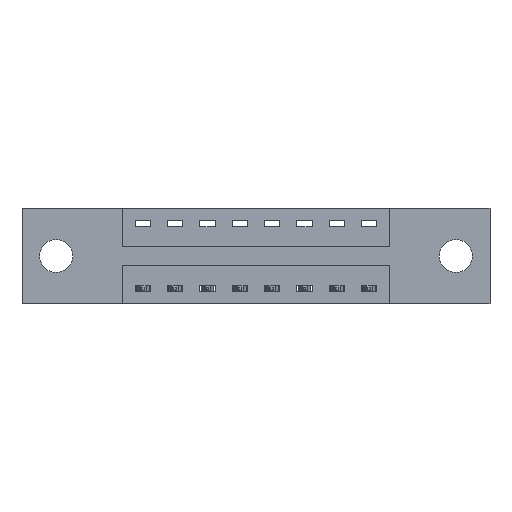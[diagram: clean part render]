
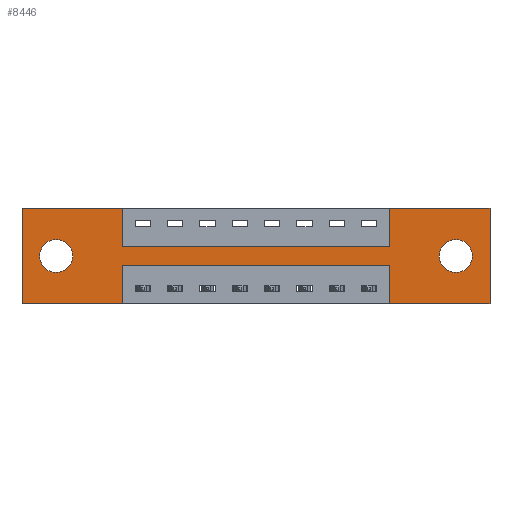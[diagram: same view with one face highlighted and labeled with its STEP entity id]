
A CAD part, front view. The second image highlights one B-rep face of the part: STEP entity #8446.
In plain terms, the highlighted planar face has unit normal (0, -1, 0).
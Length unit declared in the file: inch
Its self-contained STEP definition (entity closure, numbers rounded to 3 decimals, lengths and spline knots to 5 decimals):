
#36 = LINE ( 'NONE', #4405, #9114 ) ;
#68 = CARTESIAN_POINT ( 'NONE',  ( 0.3875, 0., -0.37 ) ) ;
#102 = VECTOR ( 'NONE', #4733, 39.37008 ) ;
#180 = VERTEX_POINT ( 'NONE', #5444 ) ;
#220 = LINE ( 'NONE', #68, #4136 ) ;
#350 = AXIS2_PLACEMENT_3D ( 'NONE', #5021, #8691, #3470 ) ;
#361 = EDGE_CURVE ( 'NONE', #2038, #2089, #7984, .T. ) ;
#451 = CARTESIAN_POINT ( 'NONE',  ( 0.1325, 0., -0.185 ) ) ;
#461 = VECTOR ( 'NONE', #2829, 39.37008 ) ;
#478 = EDGE_CURVE ( 'NONE', #9548, #180, #2171, .T. ) ;
#603 = VERTEX_POINT ( 'NONE', #5477 ) ;
#650 = EDGE_CURVE ( 'NONE', #9427, #603, #4993, .T. ) ;
#817 = CARTESIAN_POINT ( 'NONE',  ( 1.6775, 0., -0.185 ) ) ;
#1143 = VERTEX_POINT ( 'NONE', #4393 ) ;
#1163 = VERTEX_POINT ( 'NONE', #2121 ) ;
#1198 = CARTESIAN_POINT ( 'NONE',  ( 0., 0., -0.37 ) ) ;
#1335 = VECTOR ( 'NONE', #1476, 39.37008 ) ;
#1385 = CARTESIAN_POINT ( 'NONE',  ( 0., 0., 0. ) ) ;
#1429 = LINE ( 'NONE', #1385, #2047 ) ;
#1476 = DIRECTION ( 'NONE',  ( 0., 0., 1. ) ) ;
#1690 = VECTOR ( 'NONE', #2498, 39.37008 ) ;
#1725 = EDGE_LOOP ( 'NONE', ( #2457, #5234, #5663, #4398, #7138, #2356, #2877, #5528, #3506, #6196, #2540, #4841 ) ) ;
#1745 = VERTEX_POINT ( 'NONE', #7530 ) ;
#1828 = DIRECTION ( 'NONE',  ( 0., 0., -1. ) ) ;
#1904 = EDGE_CURVE ( 'NONE', #2089, #7087, #1429, .T. ) ;
#1927 = DIRECTION ( 'NONE',  ( 0., 0., 1. ) ) ;
#1958 = CARTESIAN_POINT ( 'NONE',  ( 1.6775, 0., -0.185 ) ) ;
#2038 = VERTEX_POINT ( 'NONE', #8992 ) ;
#2047 = VECTOR ( 'NONE', #7213, 39.37008 ) ;
#2089 = VERTEX_POINT ( 'NONE', #2553 ) ;
#2121 = CARTESIAN_POINT ( 'NONE',  ( 0.3875, 0., -0.37 ) ) ;
#2154 = EDGE_CURVE ( 'NONE', #180, #9548, #8745, .T. ) ;
#2171 = CIRCLE ( 'NONE', #8862, 0.064 ) ;
#2196 = DIRECTION ( 'NONE',  ( 0., -1., 0. ) ) ;
#2202 = VERTEX_POINT ( 'NONE', #2324 ) ;
#2206 = EDGE_CURVE ( 'NONE', #1143, #1745, #7455, .T. ) ;
#2324 = CARTESIAN_POINT ( 'NONE',  ( 1.81, 0., -0.37 ) ) ;
#2356 = ORIENTED_EDGE ( 'NONE', *, *, #1904, .F. ) ;
#2402 = AXIS2_PLACEMENT_3D ( 'NONE', #2970, #2196, #3796 ) ;
#2457 = ORIENTED_EDGE ( 'NONE', *, *, #4424, .F. ) ;
#2498 = DIRECTION ( 'NONE',  ( 1., 0., 0. ) ) ;
#2540 = ORIENTED_EDGE ( 'NONE', *, *, #4110, .F. ) ;
#2550 = LINE ( 'NONE', #9058, #5057 ) ;
#2553 = CARTESIAN_POINT ( 'NONE',  ( 1.4225, 0., 0. ) ) ;
#2775 = CARTESIAN_POINT ( 'NONE',  ( 1.81, 0., 0. ) ) ;
#2789 = VECTOR ( 'NONE', #8170, 39.37008 ) ;
#2829 = DIRECTION ( 'NONE',  ( 1., 0., 0. ) ) ;
#2877 = ORIENTED_EDGE ( 'NONE', *, *, #361, .F. ) ;
#2970 = CARTESIAN_POINT ( 'NONE',  ( 0., 0., -0.37 ) ) ;
#3041 = CARTESIAN_POINT ( 'NONE',  ( 1.4225, 0., -0.37 ) ) ;
#3123 = FACE_BOUND ( 'NONE', #6140, .T. ) ;
#3143 = ORIENTED_EDGE ( 'NONE', *, *, #2154, .T. ) ;
#3180 = CARTESIAN_POINT ( 'NONE',  ( 0., 0., 0. ) ) ;
#3295 = VERTEX_POINT ( 'NONE', #7139 ) ;
#3379 = LINE ( 'NONE', #6351, #6616 ) ;
#3470 = DIRECTION ( 'NONE',  ( 0., 0., 1. ) ) ;
#3506 = ORIENTED_EDGE ( 'NONE', *, *, #5926, .F. ) ;
#3557 = VECTOR ( 'NONE', #7533, 39.37008 ) ;
#3655 = FACE_OUTER_BOUND ( 'NONE', #1725, .T. ) ;
#3781 = ORIENTED_EDGE ( 'NONE', *, *, #650, .T. ) ;
#3796 = DIRECTION ( 'NONE',  ( 0., 0., -1. ) ) ;
#3813 = VERTEX_POINT ( 'NONE', #6074 ) ;
#3902 = LINE ( 'NONE', #3180, #461 ) ;
#4110 = EDGE_CURVE ( 'NONE', #4231, #3295, #5169, .T. ) ;
#4136 = VECTOR ( 'NONE', #4541, 39.37008 ) ;
#4187 = EDGE_LOOP ( 'NONE', ( #4521, #3781 ) ) ;
#4223 = VECTOR ( 'NONE', #4558, 39.37008 ) ;
#4231 = VERTEX_POINT ( 'NONE', #1198 ) ;
#4342 = CARTESIAN_POINT ( 'NONE',  ( 0.3875, 0., -0.15 ) ) ;
#4378 = CARTESIAN_POINT ( 'NONE',  ( 1.4225, 0., 0. ) ) ;
#4393 = CARTESIAN_POINT ( 'NONE',  ( 1.4225, 0., -0.22 ) ) ;
#4398 = ORIENTED_EDGE ( 'NONE', *, *, #8608, .F. ) ;
#4405 = CARTESIAN_POINT ( 'NONE',  ( 1.81, 0., 0. ) ) ;
#4424 = EDGE_CURVE ( 'NONE', #1745, #1163, #220, .T. ) ;
#4472 = VERTEX_POINT ( 'NONE', #3041 ) ;
#4521 = ORIENTED_EDGE ( 'NONE', *, *, #8176, .T. ) ;
#4541 = DIRECTION ( 'NONE',  ( 0., 0., -1. ) ) ;
#4558 = DIRECTION ( 'NONE',  ( -1., 0., 0. ) ) ;
#4733 = DIRECTION ( 'NONE',  ( -1., 0., 0. ) ) ;
#4841 = ORIENTED_EDGE ( 'NONE', *, *, #8205, .F. ) ;
#4993 = CIRCLE ( 'NONE', #350, 0.064 ) ;
#5021 = CARTESIAN_POINT ( 'NONE',  ( 0.1325, 0., -0.185 ) ) ;
#5057 = VECTOR ( 'NONE', #5363, 39.37008 ) ;
#5169 = LINE ( 'NONE', #8168, #1335 ) ;
#5234 = ORIENTED_EDGE ( 'NONE', *, *, #2206, .F. ) ;
#5308 = CARTESIAN_POINT ( 'NONE',  ( 0.3875, 0., -0.22 ) ) ;
#5363 = DIRECTION ( 'NONE',  ( -1., 0., 0. ) ) ;
#5386 = CARTESIAN_POINT ( 'NONE',  ( 0.1325, 0., -0.249 ) ) ;
#5444 = CARTESIAN_POINT ( 'NONE',  ( 1.6775, 0., -0.121 ) ) ;
#5477 = CARTESIAN_POINT ( 'NONE',  ( 0.1325, 0., -0.121 ) ) ;
#5528 = ORIENTED_EDGE ( 'NONE', *, *, #6819, .F. ) ;
#5663 = ORIENTED_EDGE ( 'NONE', *, *, #8034, .F. ) ;
#5764 = EDGE_CURVE ( 'NONE', #7087, #2202, #36, .T. ) ;
#5798 = DIRECTION ( 'NONE',  ( 0., 0., -1. ) ) ;
#5926 = EDGE_CURVE ( 'NONE', #3813, #6698, #3379, .T. ) ;
#6014 = DIRECTION ( 'NONE',  ( 0., 1., 0. ) ) ;
#6074 = CARTESIAN_POINT ( 'NONE',  ( 0.3875, 0., 0. ) ) ;
#6108 = FACE_BOUND ( 'NONE', #4187, .T. ) ;
#6140 = EDGE_LOOP ( 'NONE', ( #3143, #9020 ) ) ;
#6196 = ORIENTED_EDGE ( 'NONE', *, *, #6411, .F. ) ;
#6207 = CARTESIAN_POINT ( 'NONE',  ( 0.3875, 0., -0.15 ) ) ;
#6254 = DIRECTION ( 'NONE',  ( 0., 0., -1. ) ) ;
#6351 = CARTESIAN_POINT ( 'NONE',  ( 0.3875, 0., 0. ) ) ;
#6359 = DIRECTION ( 'NONE',  ( 0., 1., 0. ) ) ;
#6411 = EDGE_CURVE ( 'NONE', #3295, #3813, #3902, .T. ) ;
#6428 = CIRCLE ( 'NONE', #9218, 0.064 ) ;
#6616 = VECTOR ( 'NONE', #1828, 39.37008 ) ;
#6685 = LINE ( 'NONE', #6723, #3557 ) ;
#6698 = VERTEX_POINT ( 'NONE', #4342 ) ;
#6723 = CARTESIAN_POINT ( 'NONE',  ( 1.4225, 0., -0.37 ) ) ;
#6819 = EDGE_CURVE ( 'NONE', #6698, #2038, #7572, .T. ) ;
#7087 = VERTEX_POINT ( 'NONE', #2775 ) ;
#7091 = LINE ( 'NONE', #8610, #102 ) ;
#7138 = ORIENTED_EDGE ( 'NONE', *, *, #5764, .F. ) ;
#7139 = CARTESIAN_POINT ( 'NONE',  ( 0., 0., 0. ) ) ;
#7213 = DIRECTION ( 'NONE',  ( 1., 0., 0. ) ) ;
#7455 = LINE ( 'NONE', #5308, #4223 ) ;
#7530 = CARTESIAN_POINT ( 'NONE',  ( 0.3875, 0., -0.22 ) ) ;
#7533 = DIRECTION ( 'NONE',  ( 0., 0., 1. ) ) ;
#7572 = LINE ( 'NONE', #6207, #1690 ) ;
#7700 = CARTESIAN_POINT ( 'NONE',  ( 1.6775, 0., -0.249 ) ) ;
#7732 = DIRECTION ( 'NONE',  ( 0., 1., 0. ) ) ;
#7984 = LINE ( 'NONE', #4378, #2789 ) ;
#8034 = EDGE_CURVE ( 'NONE', #4472, #1143, #6685, .T. ) ;
#8168 = CARTESIAN_POINT ( 'NONE',  ( 0., 0., 0. ) ) ;
#8170 = DIRECTION ( 'NONE',  ( 0., 0., 1. ) ) ;
#8176 = EDGE_CURVE ( 'NONE', #603, #9427, #6428, .T. ) ;
#8205 = EDGE_CURVE ( 'NONE', #1163, #4231, #7091, .T. ) ;
#8446 = ADVANCED_FACE ( 'NONE', ( #3123, #6108, #3655 ), #9015, .T. ) ;
#8454 = AXIS2_PLACEMENT_3D ( 'NONE', #1958, #7732, #6254 ) ;
#8608 = EDGE_CURVE ( 'NONE', #2202, #4472, #2550, .T. ) ;
#8610 = CARTESIAN_POINT ( 'NONE',  ( 0., 0., -0.37 ) ) ;
#8691 = DIRECTION ( 'NONE',  ( 0., 1., 0. ) ) ;
#8745 = CIRCLE ( 'NONE', #8454, 0.064 ) ;
#8862 = AXIS2_PLACEMENT_3D ( 'NONE', #817, #6014, #8970 ) ;
#8970 = DIRECTION ( 'NONE',  ( 0., 0., -1. ) ) ;
#8992 = CARTESIAN_POINT ( 'NONE',  ( 1.4225, 0., -0.15 ) ) ;
#9015 = PLANE ( 'NONE',  #2402 ) ;
#9020 = ORIENTED_EDGE ( 'NONE', *, *, #478, .T. ) ;
#9058 = CARTESIAN_POINT ( 'NONE',  ( 0., 0., -0.37 ) ) ;
#9114 = VECTOR ( 'NONE', #5798, 39.37008 ) ;
#9218 = AXIS2_PLACEMENT_3D ( 'NONE', #451, #6359, #1927 ) ;
#9427 = VERTEX_POINT ( 'NONE', #5386 ) ;
#9548 = VERTEX_POINT ( 'NONE', #7700 ) ;
